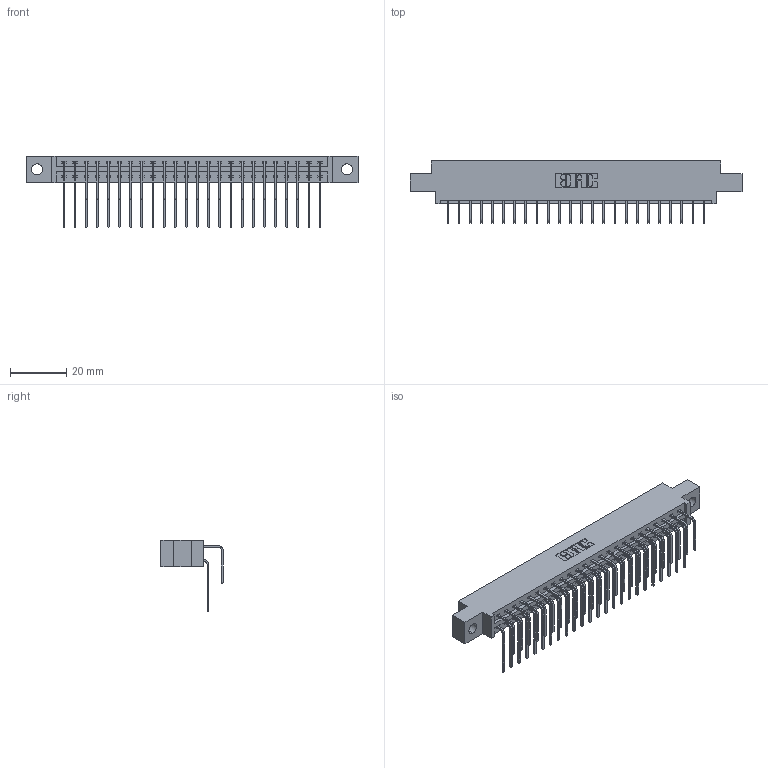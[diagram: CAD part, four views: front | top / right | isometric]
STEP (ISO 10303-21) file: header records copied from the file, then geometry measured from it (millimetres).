
FILE_DESCRIPTION (( 'STEP AP203' ), '1' );
FILE_NAME ('337-048-558-804.STEP', '2018-08-09T19:56:06', ( '' ), ( '' ), 'SwSTEP 2.0', 'SolidWorks 2016', '' );
FILE_SCHEMA (( 'CONFIG_CONTROL_DESIGN' ));
Length unit declared in the file: inch
Products named in the file (4): 345-292-001_558 Tail - 2; 337-048-558-804; 337 Part_0.170 Offset - 0.156 Dia-TH; 345-292-001_558 559 Tail - 1
Assembly tree (49 placements, depth 2):
  337-048-558-804
    337 Part_0.170 Offset - 0.156 Dia-TH
    345-292-001_558 559 Tail - 1  x24
    345-292-001_558 Tail - 2  x24
Bounding box: 118.11 x 22.17 x 25.53 mm (x, y, z)
Volume: 12279.3 mm3; surface area: 15002.5 mm2
Topology: 49 solids, 49 shells, 2806 faces, 8339 edges, 5494 vertices
Faces by surface type: plane 1994, cylinder 812
Entity records: 22855 total; most frequent: CARTESIAN_POINT 3913, ORIENTED_EDGE 3798, DIRECTION 3343, EDGE_CURVE 1899, VECTOR 1731, LINE 1731, VERTEX_POINT 1262, AXIS2_PLACEMENT_3D 806
